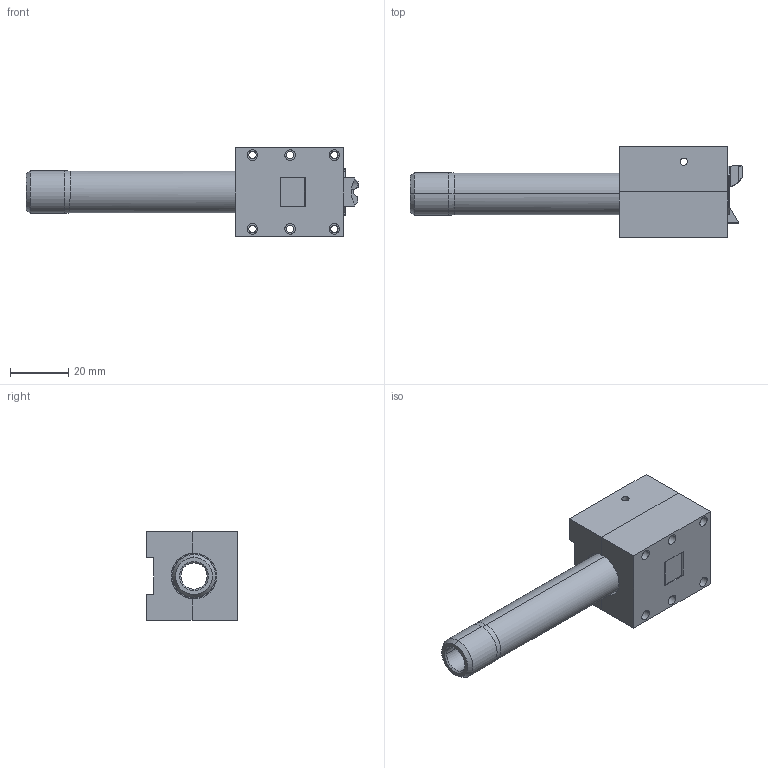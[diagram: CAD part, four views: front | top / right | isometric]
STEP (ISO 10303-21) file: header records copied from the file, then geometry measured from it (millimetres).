
FILE_DESCRIPTION (( 'STEP AP214' ), '1' );
FILE_NAME ('PPDW9 Modcat RP9 Barrel and block.STEP', '2020-12-29T19:27:58', ( '' ), ( '' ), 'SwSTEP 2.0', 'SolidWorks 2020', '' );
FILE_SCHEMA (( 'AUTOMOTIVE_DESIGN' ));
Length unit declared in the file: inch
Products named in the file (4): Barrel Block RP9 split lower; PPDW9 Modcat RP9 Barrel and block; Barrel Block RP9 split upper; Barrel RP9 Modcat modded
Assembly tree (3 placements, depth 2):
  PPDW9 Modcat RP9 Barrel and block
    Barrel RP9 Modcat modded
    Barrel Block RP9 split lower
    Barrel Block RP9 split upper
Bounding box: 114.25 x 31.24 x 30.48 mm (x, y, z)
Volume: 37042.9 mm3; surface area: 20876.7 mm2
Topology: 3 solids, 3 shells, 515 faces, 1392 edges, 900 vertices
Faces by surface type: plane 240, cylinder 127, bspline 120, sphere 13, cone 9, torus 6
Entity records: 21390 total; most frequent: CARTESIAN_POINT 8964, ORIENTED_EDGE 2764, DIRECTION 2072, EDGE_CURVE 1382, VERTEX_POINT 900, LINE 824, VECTOR 824, AXIS2_PLACEMENT_3D 624
